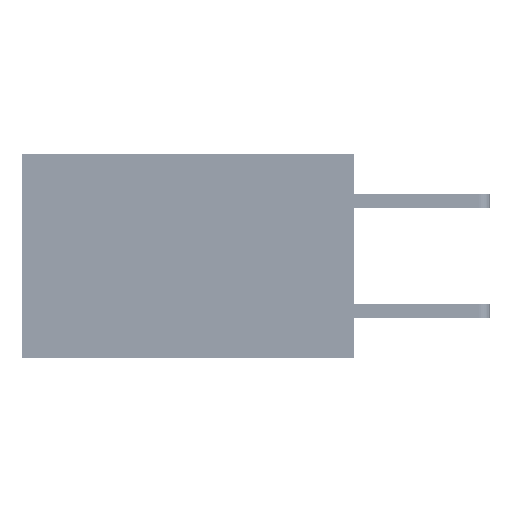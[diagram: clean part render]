
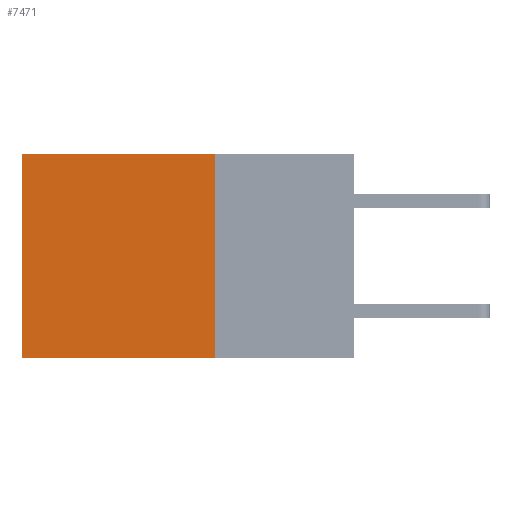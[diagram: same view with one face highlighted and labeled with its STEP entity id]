
A CAD part, left-side view. The second image highlights one B-rep face of the part: STEP entity #7471.
In plain terms, the highlighted planar face has unit normal (-1, 0, 0).
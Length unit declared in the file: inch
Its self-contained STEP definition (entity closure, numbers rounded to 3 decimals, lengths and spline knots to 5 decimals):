
#1851 = VERTEX_POINT ( 'NONE', #41417 ) ;
#2691 = DIRECTION ( 'NONE',  ( 1., 0., 0. ) ) ;
#3271 = EDGE_CURVE ( 'NONE', #1851, #6595, #6400, .T. ) ;
#3742 = VERTEX_POINT ( 'NONE', #14267 ) ;
#6127 = DIRECTION ( 'NONE',  ( 0., 0., -1. ) ) ;
#6400 = LINE ( 'NONE', #39041, #32947 ) ;
#6595 = VERTEX_POINT ( 'NONE', #42103 ) ;
#6765 = LINE ( 'NONE', #19888, #30616 ) ;
#7449 = EDGE_CURVE ( 'NONE', #1851, #17667, #6765, .T. ) ;
#7471 = ADVANCED_FACE ( 'NONE', ( #9785 ), #22275, .F. ) ;
#9785 = FACE_OUTER_BOUND ( 'NONE', #19682, .T. ) ;
#12512 = EDGE_CURVE ( 'NONE', #17667, #3742, #23614, .T. ) ;
#13229 = DIRECTION ( 'NONE',  ( 0., 0., -1. ) ) ;
#13698 = DIRECTION ( 'NONE',  ( 0., 1., 0. ) ) ;
#14267 = CARTESIAN_POINT ( 'NONE',  ( 0.2875, 0.6, -0.37 ) ) ;
#17667 = VERTEX_POINT ( 'NONE', #30580 ) ;
#17712 = DIRECTION ( 'NONE',  ( 0., 0., -1. ) ) ;
#18680 = ORIENTED_EDGE ( 'NONE', *, *, #3271, .T. ) ;
#19031 = CARTESIAN_POINT ( 'NONE',  ( 0.2875, 0.25, 0. ) ) ;
#19682 = EDGE_LOOP ( 'NONE', ( #29597, #26742, #41129, #18680 ) ) ;
#19888 = CARTESIAN_POINT ( 'NONE',  ( 0.2875, 0.25, 0. ) ) ;
#22275 = PLANE ( 'NONE',  #38833 ) ;
#23614 = LINE ( 'NONE', #30909, #28068 ) ;
#26742 = ORIENTED_EDGE ( 'NONE', *, *, #12512, .F. ) ;
#26969 = EDGE_CURVE ( 'NONE', #6595, #3742, #40890, .T. ) ;
#27415 = VECTOR ( 'NONE', #17712, 39.37008 ) ;
#28068 = VECTOR ( 'NONE', #31120, 39.37008 ) ;
#28242 = CARTESIAN_POINT ( 'NONE',  ( 0.2875, 0.6, 0. ) ) ;
#29597 = ORIENTED_EDGE ( 'NONE', *, *, #26969, .T. ) ;
#30580 = CARTESIAN_POINT ( 'NONE',  ( 0.2875, 0.25, -0.37 ) ) ;
#30616 = VECTOR ( 'NONE', #6127, 39.37008 ) ;
#30909 = CARTESIAN_POINT ( 'NONE',  ( 0.2875, 0.25, -0.37 ) ) ;
#31120 = DIRECTION ( 'NONE',  ( 0., 1., 0. ) ) ;
#32947 = VECTOR ( 'NONE', #13698, 39.37008 ) ;
#38833 = AXIS2_PLACEMENT_3D ( 'NONE', #19031, #2691, #13229 ) ;
#39041 = CARTESIAN_POINT ( 'NONE',  ( 0.2875, 0.25, 0. ) ) ;
#40890 = LINE ( 'NONE', #28242, #27415 ) ;
#41129 = ORIENTED_EDGE ( 'NONE', *, *, #7449, .F. ) ;
#41417 = CARTESIAN_POINT ( 'NONE',  ( 0.2875, 0.25, 0. ) ) ;
#42103 = CARTESIAN_POINT ( 'NONE',  ( 0.2875, 0.6, 0. ) ) ;
